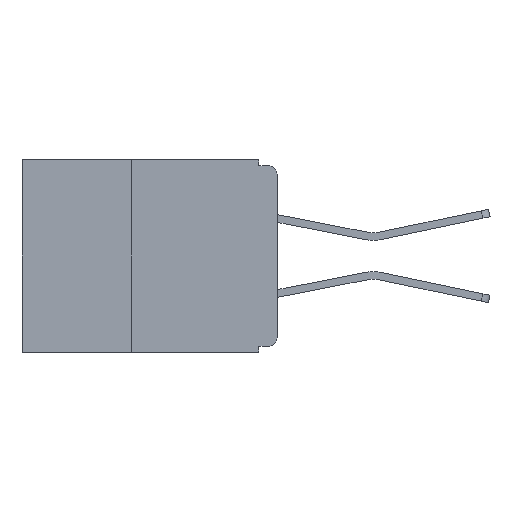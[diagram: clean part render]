
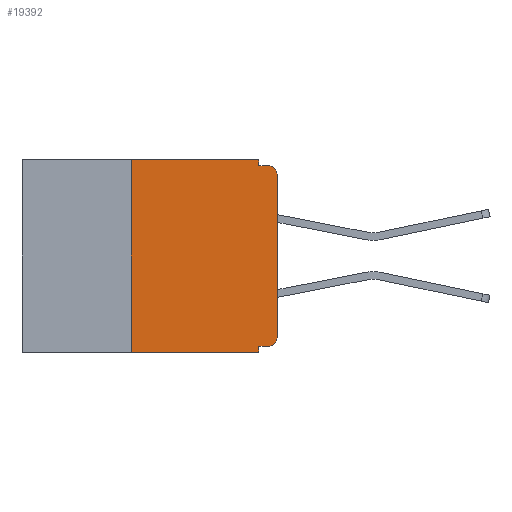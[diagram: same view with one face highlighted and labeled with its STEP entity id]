
A CAD part, left-side view. The second image highlights one B-rep face of the part: STEP entity #19392.
In plain terms, the highlighted planar face has unit normal (-1, 0, 0).
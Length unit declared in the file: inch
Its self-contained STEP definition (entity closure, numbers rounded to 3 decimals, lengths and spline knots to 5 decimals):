
#105 = CARTESIAN_POINT ( 'NONE',  ( 0., 0.031, 0. ) ) ;
#550 = EDGE_CURVE ( 'NONE', #6425, #21196, #1917, .T. ) ;
#712 = CARTESIAN_POINT ( 'NONE',  ( 0., 0.437, 0. ) ) ;
#1329 = VECTOR ( 'NONE', #1888, 39.37008 ) ;
#1417 = DIRECTION ( 'NONE',  ( -1., 0., 0. ) ) ;
#1451 = ORIENTED_EDGE ( 'NONE', *, *, #6677, .F. ) ;
#1838 = CARTESIAN_POINT ( 'NONE',  ( 0., 0., -0.025 ) ) ;
#1888 = DIRECTION ( 'NONE',  ( 0., -1., 0. ) ) ;
#1917 = LINE ( 'NONE', #7456, #1329 ) ;
#2342 = VERTEX_POINT ( 'NONE', #105 ) ;
#2408 = VECTOR ( 'NONE', #21608, 39.37008 ) ;
#2665 = DIRECTION ( 'NONE',  ( 1., 0., 0. ) ) ;
#3103 = CARTESIAN_POINT ( 'NONE',  ( 0., 0.437, 0. ) ) ;
#3549 = ORIENTED_EDGE ( 'NONE', *, *, #15808, .F. ) ;
#3899 = VERTEX_POINT ( 'NONE', #1838 ) ;
#4146 = DIRECTION ( 'NONE',  ( 0., 1., 0. ) ) ;
#5258 = LINE ( 'NONE', #6045, #18906 ) ;
#5614 = ORIENTED_EDGE ( 'NONE', *, *, #550, .F. ) ;
#5714 = EDGE_CURVE ( 'NONE', #10164, #3899, #5258, .T. ) ;
#5998 = LINE ( 'NONE', #9698, #18495 ) ;
#6045 = CARTESIAN_POINT ( 'NONE',  ( 0., 0., 0. ) ) ;
#6425 = VERTEX_POINT ( 'NONE', #9824 ) ;
#6677 = EDGE_CURVE ( 'NONE', #20616, #2342, #23119, .T. ) ;
#6824 = CARTESIAN_POINT ( 'NONE',  ( 0., 0.437, -0.33 ) ) ;
#6933 = DIRECTION ( 'NONE',  ( 0., -1., 0. ) ) ;
#7407 = VERTEX_POINT ( 'NONE', #23937 ) ;
#7456 = CARTESIAN_POINT ( 'NONE',  ( 0., 0., -0.01 ) ) ;
#7546 = CARTESIAN_POINT ( 'NONE',  ( 0., 0.015, -0.32 ) ) ;
#7715 = LINE ( 'NONE', #15413, #18132 ) ;
#7799 = VERTEX_POINT ( 'NONE', #19528 ) ;
#7863 = VERTEX_POINT ( 'NONE', #16023 ) ;
#7976 = DIRECTION ( 'NONE',  ( 0., 0., 1. ) ) ;
#8256 = ORIENTED_EDGE ( 'NONE', *, *, #5714, .T. ) ;
#8447 = VECTOR ( 'NONE', #6933, 39.37008 ) ;
#8925 = DIRECTION ( 'NONE',  ( 0., 0., -1. ) ) ;
#9423 = ORIENTED_EDGE ( 'NONE', *, *, #14582, .F. ) ;
#9698 = CARTESIAN_POINT ( 'NONE',  ( 0., 0., -0.32 ) ) ;
#9721 = DIRECTION ( 'NONE',  ( -1., 0., 0. ) ) ;
#9765 = LINE ( 'NONE', #12614, #14139 ) ;
#9824 = CARTESIAN_POINT ( 'NONE',  ( 0., 0.031, -0.01 ) ) ;
#10164 = VERTEX_POINT ( 'NONE', #20341 ) ;
#10880 = ORIENTED_EDGE ( 'NONE', *, *, #14907, .T. ) ;
#11986 = PLANE ( 'NONE',  #23798 ) ;
#12071 = EDGE_CURVE ( 'NONE', #7407, #7799, #9765, .T. ) ;
#12614 = CARTESIAN_POINT ( 'NONE',  ( 0., 0.031, -0.33 ) ) ;
#12619 = LINE ( 'NONE', #6824, #2408 ) ;
#12651 = CARTESIAN_POINT ( 'NONE',  ( 0., 0.015, -0.305 ) ) ;
#13266 = CARTESIAN_POINT ( 'NONE',  ( 0., 0.25, 0. ) ) ;
#13335 = EDGE_CURVE ( 'NONE', #7863, #7799, #12619, .T. ) ;
#14115 = VERTEX_POINT ( 'NONE', #7546 ) ;
#14139 = VECTOR ( 'NONE', #8925, 39.37008 ) ;
#14291 = VECTOR ( 'NONE', #17408, 39.37008 ) ;
#14528 = DIRECTION ( 'NONE',  ( 0., 0., -1. ) ) ;
#14582 = EDGE_CURVE ( 'NONE', #7863, #20616, #7715, .T. ) ;
#14871 = LINE ( 'NONE', #15512, #14291 ) ;
#14907 = EDGE_CURVE ( 'NONE', #14115, #10164, #19271, .T. ) ;
#15413 = CARTESIAN_POINT ( 'NONE',  ( 0., 0.25, -0.33 ) ) ;
#15512 = CARTESIAN_POINT ( 'NONE',  ( 0., 0.031, 0. ) ) ;
#15727 = DIRECTION ( 'NONE',  ( 0., 0., -1. ) ) ;
#15808 = EDGE_CURVE ( 'NONE', #2342, #6425, #14871, .T. ) ;
#15890 = EDGE_LOOP ( 'NONE', ( #8256, #21837, #5614, #3549, #1451, #9423, #23802, #21597, #20182, #10880 ) ) ;
#16023 = CARTESIAN_POINT ( 'NONE',  ( 0., 0.25, -0.33 ) ) ;
#16866 = AXIS2_PLACEMENT_3D ( 'NONE', #12651, #1417, #14528 ) ;
#17290 = DIRECTION ( 'NONE',  ( 0., 0., 1. ) ) ;
#17382 = EDGE_CURVE ( 'NONE', #3899, #21196, #18334, .T. ) ;
#17408 = DIRECTION ( 'NONE',  ( 0., 0., -1. ) ) ;
#18132 = VECTOR ( 'NONE', #17290, 39.37008 ) ;
#18334 = CIRCLE ( 'NONE', #20920, 0.015 ) ;
#18495 = VECTOR ( 'NONE', #4146, 39.37008 ) ;
#18906 = VECTOR ( 'NONE', #7976, 39.37008 ) ;
#19271 = CIRCLE ( 'NONE', #16866, 0.015 ) ;
#19392 = ADVANCED_FACE ( 'NONE', ( #23886 ), #11986, .F. ) ;
#19528 = CARTESIAN_POINT ( 'NONE',  ( 0., 0.031, -0.33 ) ) ;
#19866 = EDGE_CURVE ( 'NONE', #14115, #7407, #5998, .T. ) ;
#20182 = ORIENTED_EDGE ( 'NONE', *, *, #19866, .F. ) ;
#20341 = CARTESIAN_POINT ( 'NONE',  ( 0., 0., -0.305 ) ) ;
#20616 = VERTEX_POINT ( 'NONE', #13266 ) ;
#20816 = CARTESIAN_POINT ( 'NONE',  ( 0., 0.015, -0.025 ) ) ;
#20920 = AXIS2_PLACEMENT_3D ( 'NONE', #20816, #9721, #22655 ) ;
#21196 = VERTEX_POINT ( 'NONE', #22123 ) ;
#21597 = ORIENTED_EDGE ( 'NONE', *, *, #12071, .F. ) ;
#21608 = DIRECTION ( 'NONE',  ( 0., -1., 0. ) ) ;
#21837 = ORIENTED_EDGE ( 'NONE', *, *, #17382, .T. ) ;
#22123 = CARTESIAN_POINT ( 'NONE',  ( 0., 0.015, -0.01 ) ) ;
#22655 = DIRECTION ( 'NONE',  ( 0., 0., -1. ) ) ;
#23119 = LINE ( 'NONE', #3103, #8447 ) ;
#23798 = AXIS2_PLACEMENT_3D ( 'NONE', #712, #2665, #15727 ) ;
#23802 = ORIENTED_EDGE ( 'NONE', *, *, #13335, .T. ) ;
#23886 = FACE_OUTER_BOUND ( 'NONE', #15890, .T. ) ;
#23937 = CARTESIAN_POINT ( 'NONE',  ( 0., 0.031, -0.32 ) ) ;
